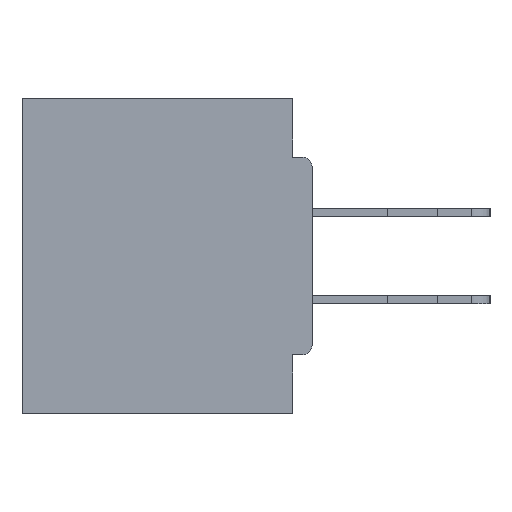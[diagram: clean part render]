
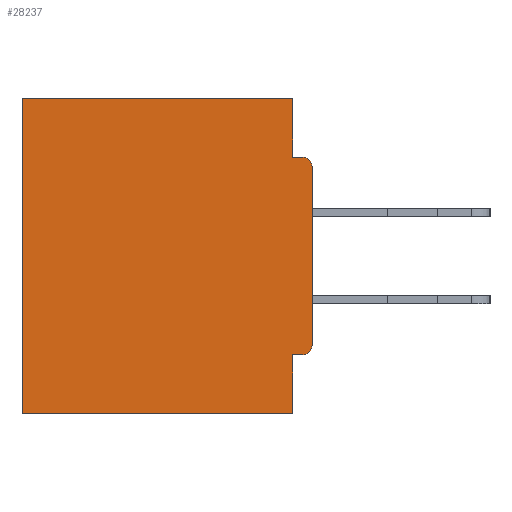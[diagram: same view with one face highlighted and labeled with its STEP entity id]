
A CAD part, left-side view. The second image highlights one B-rep face of the part: STEP entity #28237.
In plain terms, the highlighted planar face has unit normal (-1, 0, 0).
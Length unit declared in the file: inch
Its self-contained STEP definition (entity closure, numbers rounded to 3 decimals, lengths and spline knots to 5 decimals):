
#172 = CARTESIAN_POINT ( 'NONE',  ( 0.298, 0., -0.3915 ) ) ;
#525 = CARTESIAN_POINT ( 'NONE',  ( 0.298, 0., -0.0935 ) ) ;
#614 = CARTESIAN_POINT ( 'NONE',  ( 0.298, 0., 0. ) ) ;
#898 = ORIENTED_EDGE ( 'NONE', *, *, #32840, .F. ) ;
#1137 = AXIS2_PLACEMENT_3D ( 'NONE', #614, #20361, #14896 ) ;
#1539 = CARTESIAN_POINT ( 'NONE',  ( 0.298, 0., -0.4065 ) ) ;
#1859 = DIRECTION ( 'NONE',  ( 0., 0., -1. ) ) ;
#2024 = VERTEX_POINT ( 'NONE', #33344 ) ;
#2604 = VECTOR ( 'NONE', #18762, 39.37008 ) ;
#2971 = CARTESIAN_POINT ( 'NONE',  ( 0.298, 0.031, -0.4065 ) ) ;
#3498 = AXIS2_PLACEMENT_3D ( 'NONE', #17481, #28744, #11582 ) ;
#3894 = CARTESIAN_POINT ( 'NONE',  ( 0.298, 0.015, -0.4065 ) ) ;
#5644 = EDGE_CURVE ( 'NONE', #27925, #11026, #33726, .T. ) ;
#5875 = EDGE_CURVE ( 'NONE', #20167, #26321, #18669, .T. ) ;
#5878 = CARTESIAN_POINT ( 'NONE',  ( 0.298, 0.031, -0.5 ) ) ;
#5934 = VERTEX_POINT ( 'NONE', #6391 ) ;
#6151 = PLANE ( 'NONE',  #1137 ) ;
#6391 = CARTESIAN_POINT ( 'NONE',  ( 0.298, 0.031, -0.5 ) ) ;
#7499 = EDGE_CURVE ( 'NONE', #16641, #5934, #33175, .T. ) ;
#8951 = ORIENTED_EDGE ( 'NONE', *, *, #12633, .F. ) ;
#10070 = LINE ( 'NONE', #32853, #2604 ) ;
#10159 = EDGE_CURVE ( 'NONE', #15240, #2024, #12854, .T. ) ;
#10860 = VECTOR ( 'NONE', #17296, 39.37008 ) ;
#10923 = CARTESIAN_POINT ( 'NONE',  ( 0.298, 0.46, 0. ) ) ;
#11026 = VERTEX_POINT ( 'NONE', #10923 ) ;
#11582 = DIRECTION ( 'NONE',  ( 0., 0., -1. ) ) ;
#12353 = DIRECTION ( 'NONE',  ( 0., 1., 0. ) ) ;
#12633 = EDGE_CURVE ( 'NONE', #5934, #34306, #10070, .T. ) ;
#12854 = CIRCLE ( 'NONE', #31424, 0.015 ) ;
#12937 = CARTESIAN_POINT ( 'NONE',  ( 0.298, 0.031, -0.5 ) ) ;
#13790 = LINE ( 'NONE', #22173, #21297 ) ;
#14896 = DIRECTION ( 'NONE',  ( 0., 0., -1. ) ) ;
#15240 = VERTEX_POINT ( 'NONE', #35735 ) ;
#16604 = EDGE_LOOP ( 'NONE', ( #31461, #898, #31242, #30671, #23543, #8951, #29740, #34601, #18737, #31174 ) ) ;
#16641 = VERTEX_POINT ( 'NONE', #2971 ) ;
#17296 = DIRECTION ( 'NONE',  ( 0., -1., 0. ) ) ;
#17448 = EDGE_CURVE ( 'NONE', #15240, #26321, #13790, .T. ) ;
#17481 = CARTESIAN_POINT ( 'NONE',  ( 0.298, 0.015, -0.3915 ) ) ;
#17566 = LINE ( 'NONE', #1539, #30819 ) ;
#18205 = VECTOR ( 'NONE', #1859, 39.37008 ) ;
#18440 = DIRECTION ( 'NONE',  ( 0., 0., -1. ) ) ;
#18669 = CIRCLE ( 'NONE', #3498, 0.015 ) ;
#18698 = VECTOR ( 'NONE', #12353, 39.37008 ) ;
#18737 = ORIENTED_EDGE ( 'NONE', *, *, #5875, .T. ) ;
#18762 = DIRECTION ( 'NONE',  ( 0., 1., 0. ) ) ;
#20013 = FACE_OUTER_BOUND ( 'NONE', #16604, .T. ) ;
#20070 = CARTESIAN_POINT ( 'NONE',  ( 0.298, 0.46, -0.5 ) ) ;
#20167 = VERTEX_POINT ( 'NONE', #3894 ) ;
#20361 = DIRECTION ( 'NONE',  ( 1., 0., 0. ) ) ;
#21297 = VECTOR ( 'NONE', #30713, 39.37008 ) ;
#21341 = CARTESIAN_POINT ( 'NONE',  ( 0.298, 0.031, 0. ) ) ;
#22173 = CARTESIAN_POINT ( 'NONE',  ( 0.298, 0., 0. ) ) ;
#23543 = ORIENTED_EDGE ( 'NONE', *, *, #34635, .T. ) ;
#24072 = DIRECTION ( 'NONE',  ( 0., 1., 0. ) ) ;
#24291 = VECTOR ( 'NONE', #35440, 39.37008 ) ;
#26321 = VERTEX_POINT ( 'NONE', #172 ) ;
#27925 = VERTEX_POINT ( 'NONE', #21341 ) ;
#27991 = DIRECTION ( 'NONE',  ( 0., 0., -1. ) ) ;
#28237 = ADVANCED_FACE ( 'NONE', ( #20013 ), #6151, .F. ) ;
#28408 = VERTEX_POINT ( 'NONE', #32320 ) ;
#28744 = DIRECTION ( 'NONE',  ( -1., 0., 0. ) ) ;
#29280 = CARTESIAN_POINT ( 'NONE',  ( 0.298, 0., 0. ) ) ;
#29328 = EDGE_CURVE ( 'NONE', #27925, #28408, #36283, .T. ) ;
#29740 = ORIENTED_EDGE ( 'NONE', *, *, #7499, .F. ) ;
#30179 = VECTOR ( 'NONE', #27991, 39.37008 ) ;
#30567 = CARTESIAN_POINT ( 'NONE',  ( 0.298, 0.46, 0. ) ) ;
#30671 = ORIENTED_EDGE ( 'NONE', *, *, #5644, .T. ) ;
#30713 = DIRECTION ( 'NONE',  ( 0., 0., -1. ) ) ;
#30819 = VECTOR ( 'NONE', #24072, 39.37008 ) ;
#31174 = ORIENTED_EDGE ( 'NONE', *, *, #17448, .F. ) ;
#31242 = ORIENTED_EDGE ( 'NONE', *, *, #29328, .F. ) ;
#31424 = AXIS2_PLACEMENT_3D ( 'NONE', #32512, #35331, #18440 ) ;
#31461 = ORIENTED_EDGE ( 'NONE', *, *, #10159, .T. ) ;
#32320 = CARTESIAN_POINT ( 'NONE',  ( 0.298, 0.031, -0.0935 ) ) ;
#32506 = EDGE_CURVE ( 'NONE', #20167, #16641, #17566, .T. ) ;
#32512 = CARTESIAN_POINT ( 'NONE',  ( 0.298, 0.015, -0.1085 ) ) ;
#32840 = EDGE_CURVE ( 'NONE', #28408, #2024, #36073, .T. ) ;
#32853 = CARTESIAN_POINT ( 'NONE',  ( 0.298, 0., -0.5 ) ) ;
#33175 = LINE ( 'NONE', #5878, #24291 ) ;
#33344 = CARTESIAN_POINT ( 'NONE',  ( 0.298, 0.015, -0.0935 ) ) ;
#33726 = LINE ( 'NONE', #29280, #18698 ) ;
#34306 = VERTEX_POINT ( 'NONE', #20070 ) ;
#34601 = ORIENTED_EDGE ( 'NONE', *, *, #32506, .F. ) ;
#34629 = LINE ( 'NONE', #30567, #30179 ) ;
#34635 = EDGE_CURVE ( 'NONE', #11026, #34306, #34629, .T. ) ;
#35331 = DIRECTION ( 'NONE',  ( -1., 0., 0. ) ) ;
#35440 = DIRECTION ( 'NONE',  ( 0., 0., -1. ) ) ;
#35735 = CARTESIAN_POINT ( 'NONE',  ( 0.298, 0., -0.1085 ) ) ;
#36073 = LINE ( 'NONE', #525, #10860 ) ;
#36283 = LINE ( 'NONE', #12937, #18205 ) ;
